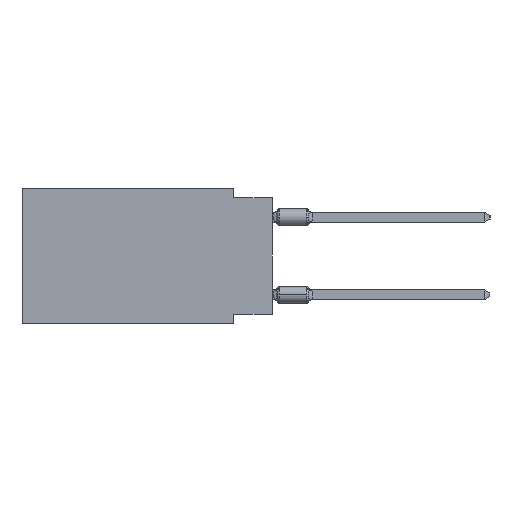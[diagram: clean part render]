
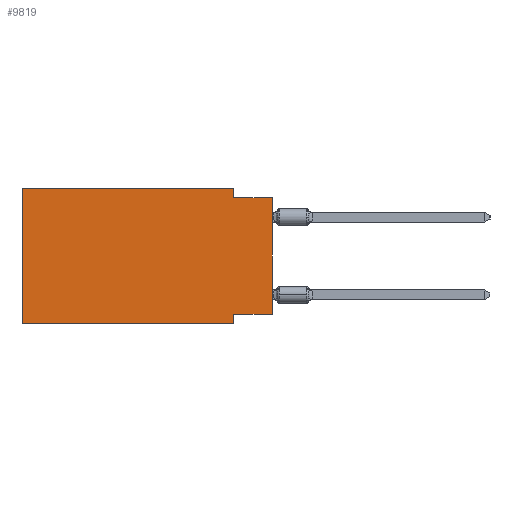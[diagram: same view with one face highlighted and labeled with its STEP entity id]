
A CAD part, left-side view. The second image highlights one B-rep face of the part: STEP entity #9819.
In plain terms, the highlighted planar face has unit normal (-1, 0, 0).
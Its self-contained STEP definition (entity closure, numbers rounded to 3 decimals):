
#569 = VERTEX_POINT ( 'NONE', #52585 ) ;
#725 = EDGE_LOOP ( 'NONE', ( #12944, #4389, #1473, #45639, #22470, #13741, #59691, #57510 ) ) ;
#975 = VECTOR ( 'NONE', #33570, 1000. ) ;
#1473 = ORIENTED_EDGE ( 'NONE', *, *, #30092, .F. ) ;
#2208 = VERTEX_POINT ( 'NONE', #48046 ) ;
#3010 = VECTOR ( 'NONE', #31706, 1000. ) ;
#4389 = ORIENTED_EDGE ( 'NONE', *, *, #41709, .F. ) ;
#5857 = LINE ( 'NONE', #25174, #3010 ) ;
#6261 = DIRECTION ( 'NONE',  ( 0., 1., 0. ) ) ;
#6459 = LINE ( 'NONE', #43505, #48162 ) ;
#6552 = CARTESIAN_POINT ( 'NONE',  ( 0., 0., -0.635 ) ) ;
#8044 = CARTESIAN_POINT ( 'NONE',  ( 0., 2.54, 0. ) ) ;
#9318 = LINE ( 'NONE', #28621, #44438 ) ;
#9819 = ADVANCED_FACE ( 'NONE', ( #20869 ), #60114, .F. ) ;
#9941 = DIRECTION ( 'NONE',  ( 0., -1., 0. ) ) ;
#10200 = CARTESIAN_POINT ( 'NONE',  ( 0., 16.383, -8.89 ) ) ;
#10690 = CARTESIAN_POINT ( 'NONE',  ( 0., 0., -8.255 ) ) ;
#12340 = VERTEX_POINT ( 'NONE', #29641 ) ;
#12578 = CARTESIAN_POINT ( 'NONE',  ( 0., 2.54, -8.89 ) ) ;
#12944 = ORIENTED_EDGE ( 'NONE', *, *, #52194, .T. ) ;
#13027 = VERTEX_POINT ( 'NONE', #10200 ) ;
#13615 = CARTESIAN_POINT ( 'NONE',  ( 0., 2.54, -8.255 ) ) ;
#13741 = ORIENTED_EDGE ( 'NONE', *, *, #46864, .T. ) ;
#15012 = CARTESIAN_POINT ( 'NONE',  ( 0., 0., -0.635 ) ) ;
#15961 = DIRECTION ( 'NONE',  ( 0., 0., 1. ) ) ;
#17132 = VECTOR ( 'NONE', #31789, 1000. ) ;
#18168 = EDGE_CURVE ( 'NONE', #13027, #40716, #19982, .T. ) ;
#18311 = AXIS2_PLACEMENT_3D ( 'NONE', #26247, #35734, #40180 ) ;
#19982 = LINE ( 'NONE', #25678, #58621 ) ;
#20080 = DIRECTION ( 'NONE',  ( 0., -1., 0. ) ) ;
#20869 = FACE_OUTER_BOUND ( 'NONE', #725, .T. ) ;
#22470 = ORIENTED_EDGE ( 'NONE', *, *, #18168, .F. ) ;
#25174 = CARTESIAN_POINT ( 'NONE',  ( 0., 16.383, -8.89 ) ) ;
#25678 = CARTESIAN_POINT ( 'NONE',  ( 0., 16.383, 0. ) ) ;
#25936 = VECTOR ( 'NONE', #20080, 1000. ) ;
#26247 = CARTESIAN_POINT ( 'NONE',  ( 0., 16.383, 0. ) ) ;
#27406 = CARTESIAN_POINT ( 'NONE',  ( 0., 16.383, 0. ) ) ;
#28505 = CARTESIAN_POINT ( 'NONE',  ( 0., 2.54, -8.89 ) ) ;
#28621 = CARTESIAN_POINT ( 'NONE',  ( 0., 0., 0. ) ) ;
#29641 = CARTESIAN_POINT ( 'NONE',  ( 0., 2.54, -0.635 ) ) ;
#30092 = EDGE_CURVE ( 'NONE', #569, #12340, #32103, .T. ) ;
#31706 = DIRECTION ( 'NONE',  ( 0., -1., 0. ) ) ;
#31789 = DIRECTION ( 'NONE',  ( 0., 0., -1. ) ) ;
#32103 = LINE ( 'NONE', #8044, #17132 ) ;
#33570 = DIRECTION ( 'NONE',  ( 0., 0., -1. ) ) ;
#34128 = EDGE_CURVE ( 'NONE', #2208, #59185, #54052, .T. ) ;
#35734 = DIRECTION ( 'NONE',  ( 1., 0., 0. ) ) ;
#36773 = VERTEX_POINT ( 'NONE', #12578 ) ;
#37815 = VERTEX_POINT ( 'NONE', #6552 ) ;
#40180 = DIRECTION ( 'NONE',  ( 0., 0., -1. ) ) ;
#40716 = VERTEX_POINT ( 'NONE', #27406 ) ;
#41704 = EDGE_CURVE ( 'NONE', #40716, #569, #6459, .T. ) ;
#41709 = EDGE_CURVE ( 'NONE', #12340, #37815, #58379, .T. ) ;
#42450 = LINE ( 'NONE', #28505, #975 ) ;
#43505 = CARTESIAN_POINT ( 'NONE',  ( 0., 16.383, 0. ) ) ;
#44438 = VECTOR ( 'NONE', #15961, 1000. ) ;
#45639 = ORIENTED_EDGE ( 'NONE', *, *, #41704, .F. ) ;
#45976 = VECTOR ( 'NONE', #6261, 1000. ) ;
#46864 = EDGE_CURVE ( 'NONE', #13027, #36773, #5857, .T. ) ;
#46996 = EDGE_CURVE ( 'NONE', #59185, #36773, #42450, .T. ) ;
#48046 = CARTESIAN_POINT ( 'NONE',  ( 0., 0., -8.255 ) ) ;
#48162 = VECTOR ( 'NONE', #9941, 1000. ) ;
#52194 = EDGE_CURVE ( 'NONE', #2208, #37815, #9318, .T. ) ;
#52585 = CARTESIAN_POINT ( 'NONE',  ( 0., 2.54, 0. ) ) ;
#54052 = LINE ( 'NONE', #10690, #45976 ) ;
#57510 = ORIENTED_EDGE ( 'NONE', *, *, #34128, .F. ) ;
#58379 = LINE ( 'NONE', #15012, #25936 ) ;
#58606 = DIRECTION ( 'NONE',  ( 0., 0., 1. ) ) ;
#58621 = VECTOR ( 'NONE', #58606, 1000. ) ;
#59185 = VERTEX_POINT ( 'NONE', #13615 ) ;
#59691 = ORIENTED_EDGE ( 'NONE', *, *, #46996, .F. ) ;
#60114 = PLANE ( 'NONE',  #18311 ) ;
